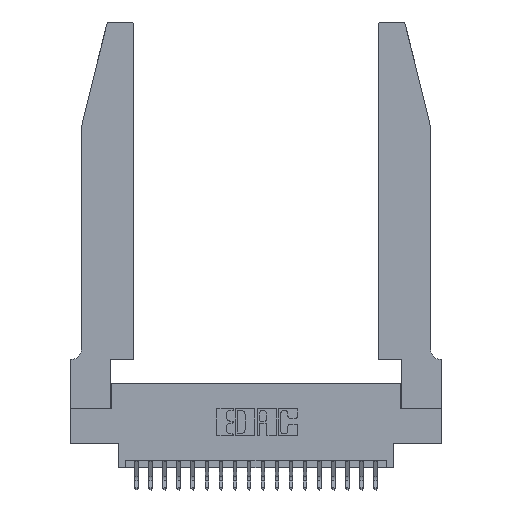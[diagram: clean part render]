
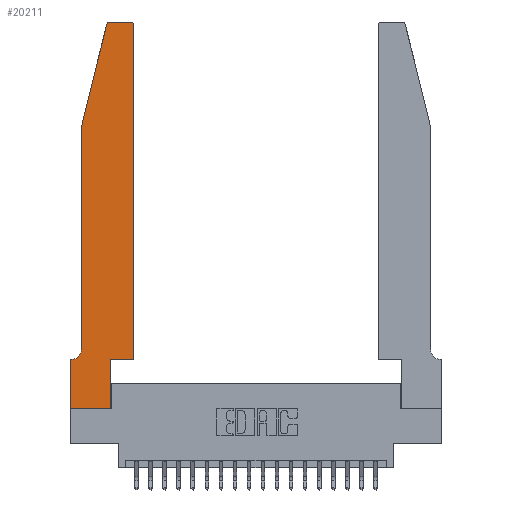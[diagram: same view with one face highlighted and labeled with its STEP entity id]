
A CAD part, top view. The second image highlights one B-rep face of the part: STEP entity #20211.
In plain terms, the highlighted planar face has unit normal (0, 0, 1).
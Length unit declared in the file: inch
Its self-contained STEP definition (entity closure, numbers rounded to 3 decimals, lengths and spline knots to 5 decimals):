
#34 = AXIS2_PLACEMENT_3D ( 'NONE', #4824, #4819, #4773 ) ;
#57 = EDGE_CURVE ( 'NONE', #14068, #9504, #7518, .T. ) ;
#134 = ORIENTED_EDGE ( 'NONE', *, *, #918, .T. ) ;
#174 = EDGE_CURVE ( 'NONE', #349, #14068, #13393, .T. ) ;
#349 = VERTEX_POINT ( 'NONE', #2523 ) ;
#356 = DIRECTION ( 'NONE',  ( 1., 0., 0. ) ) ;
#443 = ORIENTED_EDGE ( 'NONE', *, *, #13266, .T. ) ;
#552 = VECTOR ( 'NONE', #4759, 39.37008 ) ;
#711 = CARTESIAN_POINT ( 'NONE',  ( 0.2865, 0.35, 0.37 ) ) ;
#918 = EDGE_CURVE ( 'NONE', #10382, #2920, #10689, .T. ) ;
#1180 = CARTESIAN_POINT ( 'NONE',  ( 0.284, 2.72, 0.37 ) ) ;
#1614 = ORIENTED_EDGE ( 'NONE', *, *, #8204, .T. ) ;
#1977 = DIRECTION ( 'NONE',  ( 1., 0., 0. ) ) ;
#2378 = EDGE_CURVE ( 'NONE', #9504, #10382, #7292, .T. ) ;
#2523 = CARTESIAN_POINT ( 'NONE',  ( 0.2865, 0.35, 0.37 ) ) ;
#2920 = VERTEX_POINT ( 'NONE', #13399 ) ;
#3106 = DIRECTION ( 'NONE',  ( 1., 0., 0. ) ) ;
#3662 = DIRECTION ( 'NONE',  ( -0.239, -0.971, 0. ) ) ;
#4161 = EDGE_LOOP ( 'NONE', ( #134, #21165, #12754, #14018, #20972, #10530, #14368, #1614, #443, #20413, #13595, #17120 ) ) ;
#4180 = VECTOR ( 'NONE', #11054, 39.37008 ) ;
#4592 = CARTESIAN_POINT ( 'NONE',  ( 0.4505, 0.35, 0.37 ) ) ;
#4632 = CIRCLE ( 'NONE', #7298, 0.03 ) ;
#4759 = DIRECTION ( 'NONE',  ( -1., 0., 0. ) ) ;
#4764 = CARTESIAN_POINT ( 'NONE',  ( 0.4505, 0.35, 0.37 ) ) ;
#4773 = DIRECTION ( 'NONE',  ( 1., 0., 0. ) ) ;
#4819 = DIRECTION ( 'NONE',  ( 0., 0., 1. ) ) ;
#4824 = CARTESIAN_POINT ( 'NONE',  ( 0.4205, 2.72, 0.37 ) ) ;
#5266 = DIRECTION ( 'NONE',  ( -1., 0., 0. ) ) ;
#5899 = DIRECTION ( 'NONE',  ( 0., 1., 0. ) ) ;
#6564 = EDGE_CURVE ( 'NONE', #22095, #11444, #7689, .T. ) ;
#6876 = CARTESIAN_POINT ( 'NONE',  ( 0.0755, 0.35, 0.37 ) ) ;
#7273 = VERTEX_POINT ( 'NONE', #16867 ) ;
#7292 = CIRCLE ( 'NONE', #34, 0.03 ) ;
#7298 = AXIS2_PLACEMENT_3D ( 'NONE', #1180, #13579, #3106 ) ;
#7518 = LINE ( 'NONE', #11659, #15584 ) ;
#7633 = VERTEX_POINT ( 'NONE', #19781 ) ;
#7689 = LINE ( 'NONE', #21484, #8214 ) ;
#7969 = CARTESIAN_POINT ( 'NONE',  ( 0.0055, 0.42, 0.37 ) ) ;
#7972 = DIRECTION ( 'NONE',  ( 0., -1., 0. ) ) ;
#8204 = EDGE_CURVE ( 'NONE', #11444, #8400, #21348, .T. ) ;
#8214 = VECTOR ( 'NONE', #7972, 39.37008 ) ;
#8400 = VERTEX_POINT ( 'NONE', #9920 ) ;
#8687 = DIRECTION ( 'NONE',  ( 0., -1., 0. ) ) ;
#9386 = VECTOR ( 'NONE', #3662, 39.37008 ) ;
#9504 = VERTEX_POINT ( 'NONE', #9635 ) ;
#9635 = CARTESIAN_POINT ( 'NONE',  ( 0.4505, 2.72, 0.37 ) ) ;
#9689 = DIRECTION ( 'NONE',  ( -1., 0., 0. ) ) ;
#9738 = VECTOR ( 'NONE', #5266, 39.37008 ) ;
#9920 = CARTESIAN_POINT ( 'NONE',  ( 0.2865, 0., 0.37 ) ) ;
#10382 = VERTEX_POINT ( 'NONE', #12021 ) ;
#10530 = ORIENTED_EDGE ( 'NONE', *, *, #16686, .T. ) ;
#10555 = CARTESIAN_POINT ( 'NONE',  ( 0.0755, 2., 0.37 ) ) ;
#10638 = CARTESIAN_POINT ( 'NONE',  ( 0.0755, 2., 0.37 ) ) ;
#10689 = LINE ( 'NONE', #11547, #552 ) ;
#10966 = CARTESIAN_POINT ( 'NONE',  ( 0.25487, 2.72718, 0.37 ) ) ;
#11054 = DIRECTION ( 'NONE',  ( 1., 0., 0. ) ) ;
#11080 = CARTESIAN_POINT ( 'NONE',  ( 0., 0., 0.37 ) ) ;
#11199 = FACE_OUTER_BOUND ( 'NONE', #4161, .T. ) ;
#11284 = EDGE_CURVE ( 'NONE', #20242, #18004, #13948, .T. ) ;
#11332 = VECTOR ( 'NONE', #8687, 39.37008 ) ;
#11444 = VERTEX_POINT ( 'NONE', #11080 ) ;
#11547 = CARTESIAN_POINT ( 'NONE',  ( 0.2605, 2.75, 0.37 ) ) ;
#11659 = CARTESIAN_POINT ( 'NONE',  ( 0.4505, 0.35, 0.37 ) ) ;
#12009 = EDGE_CURVE ( 'NONE', #7273, #7633, #19172, .T. ) ;
#12021 = CARTESIAN_POINT ( 'NONE',  ( 0.4205, 2.75, 0.37 ) ) ;
#12557 = DIRECTION ( 'NONE',  ( 0., 0., 1. ) ) ;
#12754 = ORIENTED_EDGE ( 'NONE', *, *, #11284, .T. ) ;
#13266 = EDGE_CURVE ( 'NONE', #8400, #349, #17842, .T. ) ;
#13393 = LINE ( 'NONE', #4592, #4180 ) ;
#13399 = CARTESIAN_POINT ( 'NONE',  ( 0.284, 2.75, 0.37 ) ) ;
#13579 = DIRECTION ( 'NONE',  ( 0., 0., 1. ) ) ;
#13595 = ORIENTED_EDGE ( 'NONE', *, *, #57, .T. ) ;
#13948 = LINE ( 'NONE', #10638, #9386 ) ;
#14018 = ORIENTED_EDGE ( 'NONE', *, *, #17499, .T. ) ;
#14068 = VERTEX_POINT ( 'NONE', #4764 ) ;
#14127 = EDGE_CURVE ( 'NONE', #2920, #20242, #4632, .T. ) ;
#14186 = CARTESIAN_POINT ( 'NONE',  ( 0., 0.35, 0.37 ) ) ;
#14307 = LINE ( 'NONE', #6876, #9738 ) ;
#14368 = ORIENTED_EDGE ( 'NONE', *, *, #6564, .T. ) ;
#14648 = CARTESIAN_POINT ( 'NONE',  ( 0., 0.35, 0.37 ) ) ;
#14926 = AXIS2_PLACEMENT_3D ( 'NONE', #7969, #19813, #9689 ) ;
#15584 = VECTOR ( 'NONE', #5899, 39.37008 ) ;
#16414 = LINE ( 'NONE', #20511, #11332 ) ;
#16615 = DIRECTION ( 'NONE',  ( 0., 1., 0. ) ) ;
#16686 = EDGE_CURVE ( 'NONE', #7633, #22095, #14307, .T. ) ;
#16841 = AXIS2_PLACEMENT_3D ( 'NONE', #14186, #12557, #1977 ) ;
#16867 = CARTESIAN_POINT ( 'NONE',  ( 0.0755, 0.42, 0.37 ) ) ;
#17120 = ORIENTED_EDGE ( 'NONE', *, *, #2378, .T. ) ;
#17499 = EDGE_CURVE ( 'NONE', #18004, #7273, #16414, .T. ) ;
#17842 = LINE ( 'NONE', #711, #21684 ) ;
#18004 = VERTEX_POINT ( 'NONE', #10555 ) ;
#19172 = CIRCLE ( 'NONE', #14926, 0.07 ) ;
#19781 = CARTESIAN_POINT ( 'NONE',  ( 0.0055, 0.35, 0.37 ) ) ;
#19813 = DIRECTION ( 'NONE',  ( 0., 0., -1. ) ) ;
#20211 = ADVANCED_FACE ( 'NONE', ( #11199 ), #20878, .T. ) ;
#20242 = VERTEX_POINT ( 'NONE', #10966 ) ;
#20413 = ORIENTED_EDGE ( 'NONE', *, *, #174, .T. ) ;
#20511 = CARTESIAN_POINT ( 'NONE',  ( 0.0755, 2., 0.37 ) ) ;
#20823 = VECTOR ( 'NONE', #356, 39.37008 ) ;
#20878 = PLANE ( 'NONE',  #16841 ) ;
#20972 = ORIENTED_EDGE ( 'NONE', *, *, #12009, .T. ) ;
#21165 = ORIENTED_EDGE ( 'NONE', *, *, #14127, .T. ) ;
#21193 = CARTESIAN_POINT ( 'NONE',  ( 0., 0., 0.37 ) ) ;
#21348 = LINE ( 'NONE', #21193, #20823 ) ;
#21484 = CARTESIAN_POINT ( 'NONE',  ( 0., 0., 0.37 ) ) ;
#21684 = VECTOR ( 'NONE', #16615, 39.37008 ) ;
#22095 = VERTEX_POINT ( 'NONE', #14648 ) ;
